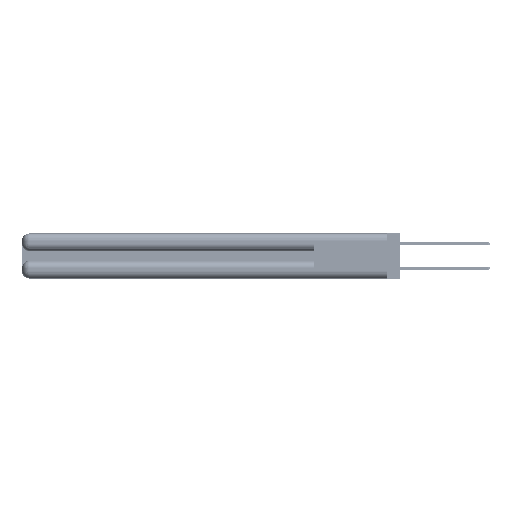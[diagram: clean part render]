
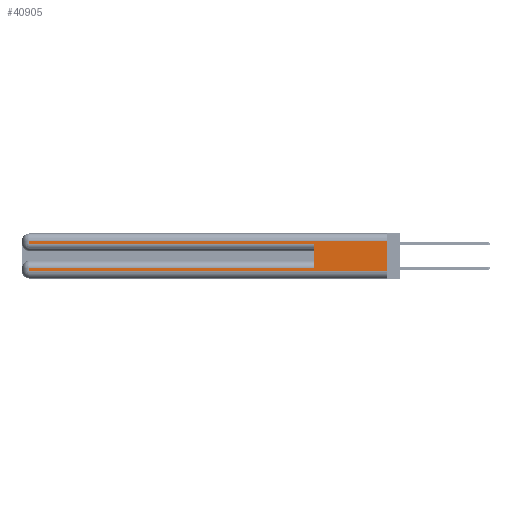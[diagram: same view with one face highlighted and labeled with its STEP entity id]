
A CAD part, left-side view. The second image highlights one B-rep face of the part: STEP entity #40905.
In plain terms, the highlighted planar face has unit normal (-1, 0, 0).
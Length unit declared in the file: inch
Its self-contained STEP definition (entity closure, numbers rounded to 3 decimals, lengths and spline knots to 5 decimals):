
#2553 = ORIENTED_EDGE ( 'NONE', *, *, #43217, .T. ) ;
#2734 = DIRECTION ( 'NONE',  ( 0., 0., -1. ) ) ;
#3024 = ORIENTED_EDGE ( 'NONE', *, *, #37649, .T. ) ;
#3853 = EDGE_CURVE ( 'NONE', #29892, #7505, #15771, .T. ) ;
#5044 = VECTOR ( 'NONE', #27131, 39.37008 ) ;
#6239 = AXIS2_PLACEMENT_3D ( 'NONE', #19932, #28585, #2734 ) ;
#6856 = CARTESIAN_POINT ( 'NONE',  ( 0., 2.94, 0.085 ) ) ;
#6941 = CARTESIAN_POINT ( 'NONE',  ( 0., 2.94, 0.285 ) ) ;
#7381 = ORIENTED_EDGE ( 'NONE', *, *, #45366, .F. ) ;
#7505 = VERTEX_POINT ( 'NONE', #17375 ) ;
#7989 = VECTOR ( 'NONE', #47920, 39.37008 ) ;
#8835 = EDGE_CURVE ( 'NONE', #21974, #24631, #18080, .T. ) ;
#13019 = EDGE_CURVE ( 'NONE', #40579, #17582, #18945, .T. ) ;
#13553 = LINE ( 'NONE', #37986, #33818 ) ;
#15771 = LINE ( 'NONE', #17621, #25888 ) ;
#16493 = DIRECTION ( 'NONE',  ( 0., 0., -1. ) ) ;
#16544 = LINE ( 'NONE', #48579, #5044 ) ;
#16754 = DIRECTION ( 'NONE',  ( 0., 1., 0. ) ) ;
#17375 = CARTESIAN_POINT ( 'NONE',  ( 0., 0., 0.06 ) ) ;
#17582 = VERTEX_POINT ( 'NONE', #18515 ) ;
#17621 = CARTESIAN_POINT ( 'NONE',  ( 0., 0., 0.06 ) ) ;
#17729 = ORIENTED_EDGE ( 'NONE', *, *, #13019, .F. ) ;
#17945 = ORIENTED_EDGE ( 'NONE', *, *, #3853, .T. ) ;
#17965 = LINE ( 'NONE', #47395, #35497 ) ;
#18080 = LINE ( 'NONE', #43583, #7989 ) ;
#18515 = CARTESIAN_POINT ( 'NONE',  ( 0., 0.6, 0.285 ) ) ;
#18945 = LINE ( 'NONE', #46639, #27695 ) ;
#19357 = DIRECTION ( 'NONE',  ( 0., -1., 0. ) ) ;
#19932 = CARTESIAN_POINT ( 'NONE',  ( 0., 0., 0.37 ) ) ;
#20177 = VECTOR ( 'NONE', #19357, 39.37008 ) ;
#21637 = CARTESIAN_POINT ( 'NONE',  ( 0., 2.94, 0.06 ) ) ;
#21888 = LINE ( 'NONE', #25609, #54905 ) ;
#21974 = VERTEX_POINT ( 'NONE', #35327 ) ;
#22207 = CARTESIAN_POINT ( 'NONE',  ( 0., 0.6, 0.085 ) ) ;
#24631 = VERTEX_POINT ( 'NONE', #6941 ) ;
#25609 = CARTESIAN_POINT ( 'NONE',  ( 0., 0., 0.085 ) ) ;
#25888 = VECTOR ( 'NONE', #26508, 39.37008 ) ;
#25951 = DIRECTION ( 'NONE',  ( 0., 1., 0. ) ) ;
#26508 = DIRECTION ( 'NONE',  ( 0., -1., 0. ) ) ;
#27131 = DIRECTION ( 'NONE',  ( 0., 0., -1. ) ) ;
#27695 = VECTOR ( 'NONE', #46833, 39.37008 ) ;
#28585 = DIRECTION ( 'NONE',  ( 1., 0., 0. ) ) ;
#29375 = ORIENTED_EDGE ( 'NONE', *, *, #8835, .T. ) ;
#29892 = VERTEX_POINT ( 'NONE', #21637 ) ;
#30398 = EDGE_CURVE ( 'NONE', #49408, #21974, #17965, .T. ) ;
#31006 = ORIENTED_EDGE ( 'NONE', *, *, #30398, .T. ) ;
#33818 = VECTOR ( 'NONE', #16493, 39.37008 ) ;
#35327 = CARTESIAN_POINT ( 'NONE',  ( 0., 2.94, 0.31 ) ) ;
#35497 = VECTOR ( 'NONE', #25951, 39.37008 ) ;
#35615 = FACE_OUTER_BOUND ( 'NONE', #52753, .T. ) ;
#36528 = CARTESIAN_POINT ( 'NONE',  ( 0., 0., 0.31 ) ) ;
#37649 = EDGE_CURVE ( 'NONE', #40579, #50113, #21888, .T. ) ;
#37986 = CARTESIAN_POINT ( 'NONE',  ( 0., 2.94, 0.37 ) ) ;
#40579 = VERTEX_POINT ( 'NONE', #22207 ) ;
#40905 = ADVANCED_FACE ( 'NONE', ( #35615 ), #54366, .F. ) ;
#41550 = ORIENTED_EDGE ( 'NONE', *, *, #54593, .T. ) ;
#43040 = LINE ( 'NONE', #49471, #20177 ) ;
#43217 = EDGE_CURVE ( 'NONE', #24631, #17582, #43040, .T. ) ;
#43583 = CARTESIAN_POINT ( 'NONE',  ( 0., 2.94, 0.37 ) ) ;
#45366 = EDGE_CURVE ( 'NONE', #49408, #7505, #16544, .T. ) ;
#46639 = CARTESIAN_POINT ( 'NONE',  ( 0., 0.6, 0.145 ) ) ;
#46833 = DIRECTION ( 'NONE',  ( 0., 0., 1. ) ) ;
#47395 = CARTESIAN_POINT ( 'NONE',  ( 0., 0., 0.31 ) ) ;
#47920 = DIRECTION ( 'NONE',  ( 0., 0., -1. ) ) ;
#48579 = CARTESIAN_POINT ( 'NONE',  ( 0., 0., 0.37 ) ) ;
#49408 = VERTEX_POINT ( 'NONE', #36528 ) ;
#49471 = CARTESIAN_POINT ( 'NONE',  ( 0., 0., 0.285 ) ) ;
#50113 = VERTEX_POINT ( 'NONE', #6856 ) ;
#52753 = EDGE_LOOP ( 'NONE', ( #7381, #31006, #29375, #2553, #17729, #3024, #41550, #17945 ) ) ;
#54366 = PLANE ( 'NONE',  #6239 ) ;
#54593 = EDGE_CURVE ( 'NONE', #50113, #29892, #13553, .T. ) ;
#54905 = VECTOR ( 'NONE', #16754, 39.37008 ) ;
